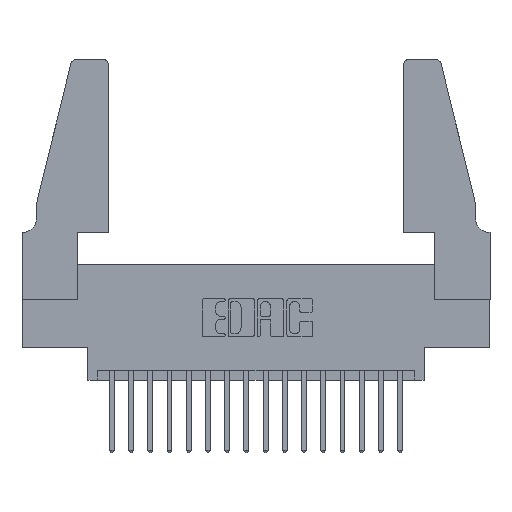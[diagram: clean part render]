
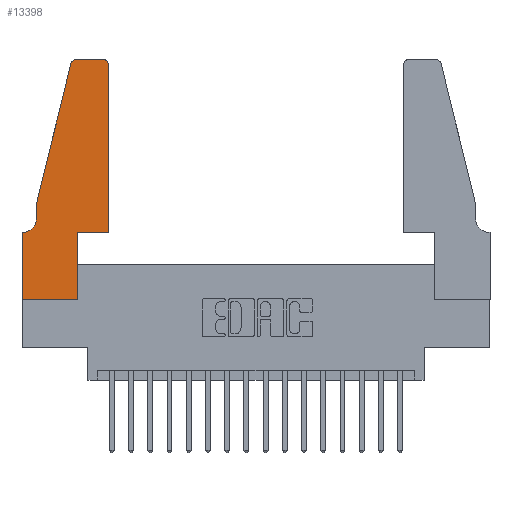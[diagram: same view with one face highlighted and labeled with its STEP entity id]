
A CAD part, top view. The second image highlights one B-rep face of the part: STEP entity #13398.
In plain terms, the highlighted planar face has unit normal (0, 0, 1).
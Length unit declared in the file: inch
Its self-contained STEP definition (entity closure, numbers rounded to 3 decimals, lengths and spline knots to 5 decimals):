
#11 = DIRECTION ( 'NONE',  ( -1., 0., 0. ) ) ;
#304 = EDGE_CURVE ( 'NONE', #981, #16631, #3019, .T. ) ;
#497 = EDGE_LOOP ( 'NONE', ( #14253, #16098, #3419, #5226, #18103, #16449, #16151, #4492, #7044, #5349, #12917, #3340 ) ) ;
#867 = LINE ( 'NONE', #5486, #12442 ) ;
#981 = VERTEX_POINT ( 'NONE', #8456 ) ;
#993 = EDGE_CURVE ( 'NONE', #13820, #13893, #1897, .T. ) ;
#1083 = DIRECTION ( 'NONE',  ( 0., 0., 1. ) ) ;
#1132 = DIRECTION ( 'NONE',  ( 0., 1., 0. ) ) ;
#1338 = VERTEX_POINT ( 'NONE', #13733 ) ;
#1366 = VECTOR ( 'NONE', #10276, 39.37008 ) ;
#1372 = LINE ( 'NONE', #6016, #12953 ) ;
#1576 = PLANE ( 'NONE',  #3009 ) ;
#1745 = DIRECTION ( 'NONE',  ( 0., 0., 1. ) ) ;
#1897 = LINE ( 'NONE', #17013, #3888 ) ;
#2110 = LINE ( 'NONE', #5560, #11675 ) ;
#2505 = CIRCLE ( 'NONE', #7464, 0.07 ) ;
#3009 = AXIS2_PLACEMENT_3D ( 'NONE', #4670, #14428, #10209 ) ;
#3019 = LINE ( 'NONE', #16491, #15490 ) ;
#3180 = VERTEX_POINT ( 'NONE', #11871 ) ;
#3198 = VERTEX_POINT ( 'NONE', #13144 ) ;
#3240 = CARTESIAN_POINT ( 'NONE',  ( 0.0755, 0.5, 0.37 ) ) ;
#3340 = ORIENTED_EDGE ( 'NONE', *, *, #9118, .T. ) ;
#3419 = ORIENTED_EDGE ( 'NONE', *, *, #14966, .T. ) ;
#3888 = VECTOR ( 'NONE', #11, 39.37008 ) ;
#4031 = EDGE_CURVE ( 'NONE', #10264, #3198, #5142, .T. ) ;
#4049 = CARTESIAN_POINT ( 'NONE',  ( 0.284, 1.22, 0.37 ) ) ;
#4492 = ORIENTED_EDGE ( 'NONE', *, *, #16043, .T. ) ;
#4657 = CARTESIAN_POINT ( 'NONE',  ( 0.4505, 0.35, 0.37 ) ) ;
#4670 = CARTESIAN_POINT ( 'NONE',  ( 0., 0.35, 0.37 ) ) ;
#4925 = CARTESIAN_POINT ( 'NONE',  ( 0.0755, 0.5, 0.37 ) ) ;
#5142 = LINE ( 'NONE', #3240, #1366 ) ;
#5226 = ORIENTED_EDGE ( 'NONE', *, *, #4031, .T. ) ;
#5349 = ORIENTED_EDGE ( 'NONE', *, *, #304, .T. ) ;
#5486 = CARTESIAN_POINT ( 'NONE',  ( 0.2865, 0.35, 0.37 ) ) ;
#5560 = CARTESIAN_POINT ( 'NONE',  ( 0., 0., 0.37 ) ) ;
#6016 = CARTESIAN_POINT ( 'NONE',  ( 0.0755, 0.5, 0.37 ) ) ;
#6863 = CARTESIAN_POINT ( 'NONE',  ( 0.284, 1.25, 0.37 ) ) ;
#7001 = EDGE_CURVE ( 'NONE', #13893, #11784, #2110, .T. ) ;
#7044 = ORIENTED_EDGE ( 'NONE', *, *, #10977, .T. ) ;
#7464 = AXIS2_PLACEMENT_3D ( 'NONE', #8817, #10304, #11886 ) ;
#7532 = VECTOR ( 'NONE', #16398, 39.37008 ) ;
#7599 = LINE ( 'NONE', #14578, #14255 ) ;
#7965 = VERTEX_POINT ( 'NONE', #15274 ) ;
#8456 = CARTESIAN_POINT ( 'NONE',  ( 0.2865, 0.35, 0.37 ) ) ;
#8817 = CARTESIAN_POINT ( 'NONE',  ( 0.0055, 0.42, 0.37 ) ) ;
#8872 = DIRECTION ( 'NONE',  ( -0.239, -0.971, 0. ) ) ;
#9118 = EDGE_CURVE ( 'NONE', #7965, #1338, #17152, .T. ) ;
#9323 = CIRCLE ( 'NONE', #12614, 0.03 ) ;
#9485 = VERTEX_POINT ( 'NONE', #6863 ) ;
#10202 = VERTEX_POINT ( 'NONE', #16185 ) ;
#10209 = DIRECTION ( 'NONE',  ( 1., 0., 0. ) ) ;
#10264 = VERTEX_POINT ( 'NONE', #4925 ) ;
#10276 = DIRECTION ( 'NONE',  ( 0., -1., 0. ) ) ;
#10304 = DIRECTION ( 'NONE',  ( 0., 0., -1. ) ) ;
#10362 = EDGE_CURVE ( 'NONE', #9485, #10202, #9323, .T. ) ;
#10977 = EDGE_CURVE ( 'NONE', #3180, #981, #867, .T. ) ;
#11039 = DIRECTION ( 'NONE',  ( 1., 0., 0. ) ) ;
#11329 = LINE ( 'NONE', #17800, #7532 ) ;
#11474 = DIRECTION ( 'NONE',  ( 0., -1., 0. ) ) ;
#11675 = VECTOR ( 'NONE', #11474, 39.37008 ) ;
#11784 = VERTEX_POINT ( 'NONE', #16251 ) ;
#11871 = CARTESIAN_POINT ( 'NONE',  ( 0.2865, 0., 0.37 ) ) ;
#11886 = DIRECTION ( 'NONE',  ( -1., 0., 0. ) ) ;
#12442 = VECTOR ( 'NONE', #1132, 39.37008 ) ;
#12614 = AXIS2_PLACEMENT_3D ( 'NONE', #4049, #1083, #11039 ) ;
#12917 = ORIENTED_EDGE ( 'NONE', *, *, #17865, .T. ) ;
#12953 = VECTOR ( 'NONE', #8872, 39.37008 ) ;
#13003 = CARTESIAN_POINT ( 'NONE',  ( 0.4205, 1.22, 0.37 ) ) ;
#13144 = CARTESIAN_POINT ( 'NONE',  ( 0.0755, 0.42, 0.37 ) ) ;
#13398 = ADVANCED_FACE ( 'NONE', ( #18322 ), #1576, .T. ) ;
#13733 = CARTESIAN_POINT ( 'NONE',  ( 0.4205, 1.25, 0.37 ) ) ;
#13820 = VERTEX_POINT ( 'NONE', #17843 ) ;
#13893 = VERTEX_POINT ( 'NONE', #16397 ) ;
#14253 = ORIENTED_EDGE ( 'NONE', *, *, #15431, .T. ) ;
#14255 = VECTOR ( 'NONE', #17341, 39.37008 ) ;
#14339 = AXIS2_PLACEMENT_3D ( 'NONE', #13003, #1745, #17309 ) ;
#14428 = DIRECTION ( 'NONE',  ( 0., 0., 1. ) ) ;
#14578 = CARTESIAN_POINT ( 'NONE',  ( 0., 0., 0.37 ) ) ;
#14966 = EDGE_CURVE ( 'NONE', #10202, #10264, #1372, .T. ) ;
#15274 = CARTESIAN_POINT ( 'NONE',  ( 0.4505, 1.22, 0.37 ) ) ;
#15431 = EDGE_CURVE ( 'NONE', #1338, #9485, #17573, .T. ) ;
#15490 = VECTOR ( 'NONE', #16677, 39.37008 ) ;
#15748 = EDGE_CURVE ( 'NONE', #3198, #13820, #2505, .T. ) ;
#16043 = EDGE_CURVE ( 'NONE', #11784, #3180, #7599, .T. ) ;
#16098 = ORIENTED_EDGE ( 'NONE', *, *, #10362, .T. ) ;
#16151 = ORIENTED_EDGE ( 'NONE', *, *, #7001, .T. ) ;
#16185 = CARTESIAN_POINT ( 'NONE',  ( 0.25487, 1.22718, 0.37 ) ) ;
#16251 = CARTESIAN_POINT ( 'NONE',  ( 0., 0., 0.37 ) ) ;
#16397 = CARTESIAN_POINT ( 'NONE',  ( 0., 0.35, 0.37 ) ) ;
#16398 = DIRECTION ( 'NONE',  ( 0., 1., 0. ) ) ;
#16449 = ORIENTED_EDGE ( 'NONE', *, *, #993, .T. ) ;
#16491 = CARTESIAN_POINT ( 'NONE',  ( 0.4505, 0.35, 0.37 ) ) ;
#16631 = VERTEX_POINT ( 'NONE', #4657 ) ;
#16677 = DIRECTION ( 'NONE',  ( 1., 0., 0. ) ) ;
#17013 = CARTESIAN_POINT ( 'NONE',  ( 0.0755, 0.35, 0.37 ) ) ;
#17152 = CIRCLE ( 'NONE', #14339, 0.03 ) ;
#17309 = DIRECTION ( 'NONE',  ( 1., 0., 0. ) ) ;
#17341 = DIRECTION ( 'NONE',  ( 1., 0., 0. ) ) ;
#17356 = VECTOR ( 'NONE', #17756, 39.37008 ) ;
#17573 = LINE ( 'NONE', #17622, #17356 ) ;
#17622 = CARTESIAN_POINT ( 'NONE',  ( 0.2605, 1.25, 0.37 ) ) ;
#17756 = DIRECTION ( 'NONE',  ( -1., 0., 0. ) ) ;
#17800 = CARTESIAN_POINT ( 'NONE',  ( 0.4505, 0.35, 0.37 ) ) ;
#17843 = CARTESIAN_POINT ( 'NONE',  ( 0.0055, 0.35, 0.37 ) ) ;
#17865 = EDGE_CURVE ( 'NONE', #16631, #7965, #11329, .T. ) ;
#18103 = ORIENTED_EDGE ( 'NONE', *, *, #15748, .T. ) ;
#18322 = FACE_OUTER_BOUND ( 'NONE', #497, .T. ) ;
